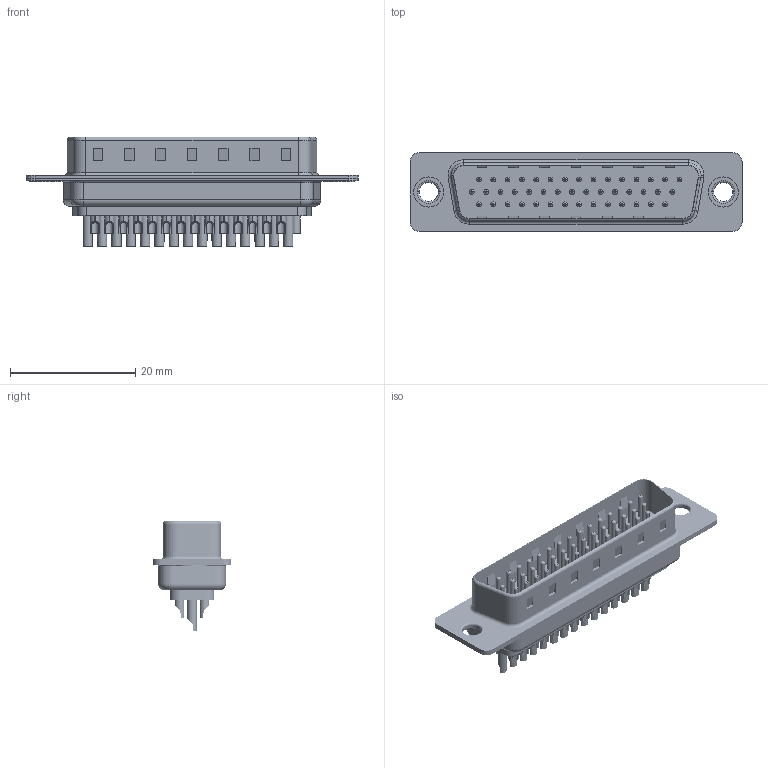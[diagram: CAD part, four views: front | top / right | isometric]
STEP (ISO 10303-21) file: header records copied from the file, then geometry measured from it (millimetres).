
FILE_DESCRIPTION (( 'STEP AP203' ), '1' );
FILE_NAME ('637-044-632-241.STEP', '2020-07-18T03:12:00', ( '' ), ( '' ), 'SwSTEP 2.0', 'SolidWorks 2020', '' );
FILE_SCHEMA (( 'CONFIG_CONTROL_DESIGN' ));
Length unit declared in the file: millimetre
Products named in the file (8): 637 Shell Rear_44 Contacts; 637-044-632-241; 637 Thru Hole Rivet; 637 Shell Front_44 Contacts; 637 Housing_44 Contacts; 637 Contact Row 2_32; 637 Contact Row 1_32; 637 Contact Row 3_32
Assembly tree (49 placements, depth 2):
  637-044-632-241
    637 Housing_44 Contacts
    637 Shell Front_44 Contacts
    637 Shell Rear_44 Contacts
    637 Contact Row 1_32  x15
    637 Contact Row 2_32  x15
    637 Contact Row 3_32  x14
    637 Thru Hole Rivet  x2
Bounding box: 53 x 12.6 x 17.55 mm (x, y, z)
Volume: 2635.4 mm3; surface area: 10285 mm2
Topology: 49 solids, 49 shells, 3166 faces, 8091 edges, 5122 vertices
Faces by surface type: cylinder 1397, torus 982, plane 787
Entity records: 27736 total; most frequent: DIRECTION 4891, CARTESIAN_POINT 4483, ORIENTED_EDGE 4130, EDGE_CURVE 2065, AXIS2_PLACEMENT_3D 1975, VERTEX_POINT 1326, EDGE_LOOP 1077, CIRCLE 1073
